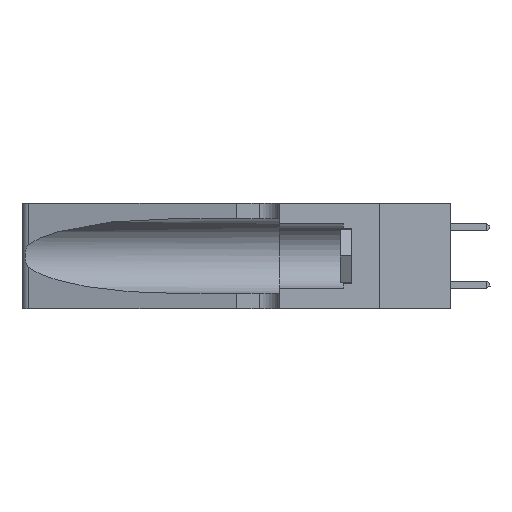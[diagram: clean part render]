
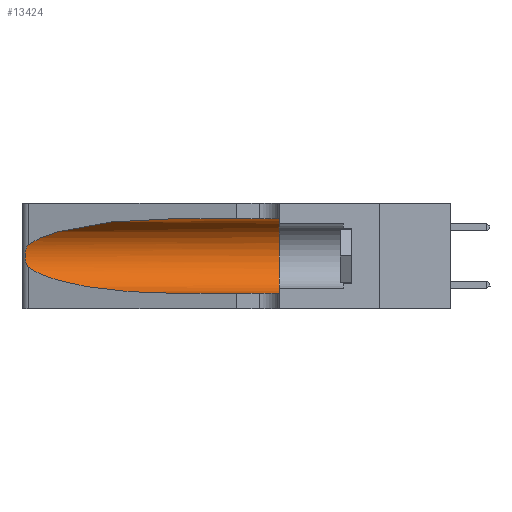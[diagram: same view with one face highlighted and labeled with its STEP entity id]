
A CAD part, left-side view. The second image highlights one B-rep face of the part: STEP entity #13424.
In plain terms, the highlighted cylindrical face has radius 3.308 mm (diameter 6.617 mm), a partial arc.
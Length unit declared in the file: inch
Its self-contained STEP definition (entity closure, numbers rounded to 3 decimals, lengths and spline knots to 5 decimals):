
#427 = CARTESIAN_POINT ( 'NONE',  ( 0.26018, 1.23835, 0.19895 ) ) ;
#2069 = ORIENTED_EDGE ( 'NONE', *, *, #15396, .F. ) ;
#2346 = CARTESIAN_POINT ( 'NONE',  ( 0.25487, 1.22718, 0.22369 ) ) ;
#3490 = CARTESIAN_POINT ( 'NONE',  ( 0.26075, 1.23896, 0.178 ) ) ;
#3949 = B_SPLINE_CURVE_WITH_KNOTS ( 'NONE', 3,
 ( #12381, #33062, #15370, #36014, #18378, #427, #21346, #3490, #24275, #6493, #27244, #9545, #30256, #12506 ),
 .UNSPECIFIED., .F., .F.,
 ( 4, 2, 2, 2, 2, 2, 4 ),
 ( 0., 0.00027, 0.00053, 0.00107, 0.0016, 0.00187, 0.00214 ),
 .UNSPECIFIED. ) ;
#4098 = CYLINDRICAL_SURFACE ( 'NONE', #31432, 0.13025 ) ;
#5398 = DIRECTION ( 'NONE',  ( 0., -1., 0. ) ) ;
#6035 = CARTESIAN_POINT ( 'NONE',  ( 0.18966, 0.96281, 0.05475 ) ) ;
#6493 = CARTESIAN_POINT ( 'NONE',  ( 0.25856, 1.23593, 0.16098 ) ) ;
#9225 = AXIS2_PLACEMENT_3D ( 'NONE', #27872, #10150, #30862 ) ;
#9545 = CARTESIAN_POINT ( 'NONE',  ( 0.25639, 1.23186, 0.15144 ) ) ;
#9634 = DIRECTION ( 'NONE',  ( 0., -1., 0. ) ) ;
#10150 = DIRECTION ( 'NONE',  ( 0., 1., 0. ) ) ;
#10249 = CARTESIAN_POINT ( 'NONE',  ( 0.1305, 0.35, 0.31525 ) ) ;
#10934 = CARTESIAN_POINT ( 'NONE',  ( 0.25487, 1.22718, 0.14631 ) ) ;
#12345 = ORIENTED_EDGE ( 'NONE', *, *, #25570, .T. ) ;
#12381 = CARTESIAN_POINT ( 'NONE',  ( 0.25487, 1.22718, 0.22369 ) ) ;
#12506 = CARTESIAN_POINT ( 'NONE',  ( 0.25487, 1.22718, 0.14631 ) ) ;
#13282 = VERTEX_POINT ( 'NONE', #10934 ) ;
#13424 = ADVANCED_FACE ( 'NONE', ( #27826 ), #4098, .F. ) ;
#13520 = LINE ( 'NONE', #27332, #29266 ) ;
#14432 = CARTESIAN_POINT ( 'NONE',  ( 0.1305, 1.61858, 0.185 ) ) ;
#14441 = DIRECTION ( 'NONE',  ( 0., -1., 0. ) ) ;
#14915 = CARTESIAN_POINT ( 'NONE',  ( 0.25487, 1.22718, 0.14631 ) ) ;
#15184 = VECTOR ( 'NONE', #14441, 39.37008 ) ;
#15370 = CARTESIAN_POINT ( 'NONE',  ( 0.25639, 1.23184, 0.21858 ) ) ;
#15396 = EDGE_CURVE ( 'NONE', #36557, #24557, #30006, .T. ) ;
#16826 = VERTEX_POINT ( 'NONE', #26480 ) ;
#16879 = CARTESIAN_POINT ( 'NONE',  ( 0.25487, 1.22718, 0.22369 ) ) ;
#17233 = CARTESIAN_POINT ( 'NONE',  ( 0.18966, 0.96281, 0.31525 ) ) ;
#17475 = ORIENTED_EDGE ( 'NONE', *, *, #31142, .T. ) ;
#17672 = CARTESIAN_POINT ( 'NONE',  ( 0.1305, 0.72297, 0.31525 ) ) ;
#17927 = CARTESIAN_POINT ( 'NONE',  ( 0.2373, 1.15595, 0.08982 ) ) ;
#18093 = CIRCLE ( 'NONE', #9225, 0.13025 ) ;
#18378 = CARTESIAN_POINT ( 'NONE',  ( 0.25854, 1.2359, 0.20912 ) ) ;
#20234 = CARTESIAN_POINT ( 'NONE',  ( 0.2373, 1.15595, 0.28018 ) ) ;
#21346 = CARTESIAN_POINT ( 'NONE',  ( 0.26075, 1.23896, 0.19203 ) ) ;
#23474 = ORIENTED_EDGE ( 'NONE', *, *, #36208, .F. ) ;
#23916 = ORIENTED_EDGE ( 'NONE', *, *, #31673, .T. ) ;
#24275 = CARTESIAN_POINT ( 'NONE',  ( 0.26017, 1.23833, 0.17102 ) ) ;
#24557 = VERTEX_POINT ( 'NONE', #10249 ) ;
#25570 = EDGE_CURVE ( 'NONE', #30898, #13282, #3949, .T. ) ;
#25694 = VERTEX_POINT ( 'NONE', #30759 ) ;
#26480 = CARTESIAN_POINT ( 'NONE',  ( 0.1305, 0.35, 0.05475 ) ) ;
#26792 = CARTESIAN_POINT ( 'NONE',  ( 0.1305, 0.72297, 0.05475 ) ) ;
#27244 = CARTESIAN_POINT ( 'NONE',  ( 0.25789, 1.23486, 0.15765 ) ) ;
#27266 = EDGE_CURVE ( 'NONE', #25694, #16826, #13520, .T. ) ;
#27332 = CARTESIAN_POINT ( 'NONE',  ( 0.1305, 1.61858, 0.05475 ) ) ;
#27826 = FACE_OUTER_BOUND ( 'NONE', #36133, .T. ) ;
#27872 = CARTESIAN_POINT ( 'NONE',  ( 0.1305, 0.35, 0.185 ) ) ;
#28980 = CARTESIAN_POINT ( 'NONE',  ( 0.1305, 0.72297, 0.31525 ) ) ;
#28998 =( BOUNDED_CURVE ( )  B_SPLINE_CURVE ( 3, ( #14915, #17927, #6035, #26792 ),
 .UNSPECIFIED., .F., .T. ) 
 B_SPLINE_CURVE_WITH_KNOTS ( ( 4, 4 ),
 ( 3.44316, 4.71239 ),
 .UNSPECIFIED. ) 
 CURVE ( )  GEOMETRIC_REPRESENTATION_ITEM ( )  RATIONAL_B_SPLINE_CURVE ( ( 1., 0.87, 0.87, 1. ) ) 
 REPRESENTATION_ITEM ( '' )  );
#29266 = VECTOR ( 'NONE', #9634, 39.37008 ) ;
#29945 = ORIENTED_EDGE ( 'NONE', *, *, #27266, .T. ) ;
#30006 = LINE ( 'NONE', #32159, #15184 ) ;
#30256 = CARTESIAN_POINT ( 'NONE',  ( 0.25555, 1.22993, 0.14849 ) ) ;
#30759 = CARTESIAN_POINT ( 'NONE',  ( 0.1305, 0.72297, 0.05475 ) ) ;
#30862 = DIRECTION ( 'NONE',  ( 0., 0., 1. ) ) ;
#30898 = VERTEX_POINT ( 'NONE', #16879 ) ;
#31142 = EDGE_CURVE ( 'NONE', #13282, #25694, #28998, .T. ) ;
#31432 = AXIS2_PLACEMENT_3D ( 'NONE', #14432, #5398, #32147 ) ;
#31673 = EDGE_CURVE ( 'NONE', #36557, #30898, #36507, .T. ) ;
#32147 = DIRECTION ( 'NONE',  ( 0., 0., -1. ) ) ;
#32159 = CARTESIAN_POINT ( 'NONE',  ( 0.1305, 1.61858, 0.31525 ) ) ;
#33062 = CARTESIAN_POINT ( 'NONE',  ( 0.25555, 1.22994, 0.2215 ) ) ;
#36014 = CARTESIAN_POINT ( 'NONE',  ( 0.25787, 1.23484, 0.2124 ) ) ;
#36133 = EDGE_LOOP ( 'NONE', ( #23916, #12345, #17475, #29945, #23474, #2069 ) ) ;
#36208 = EDGE_CURVE ( 'NONE', #24557, #16826, #18093, .T. ) ;
#36507 =( BOUNDED_CURVE ( )  B_SPLINE_CURVE ( 3, ( #28980, #17233, #20234, #2346 ),
 .UNSPECIFIED., .F., .T. ) 
 B_SPLINE_CURVE_WITH_KNOTS ( ( 4, 4 ),
 ( 1.5708, 2.84003 ),
 .UNSPECIFIED. ) 
 CURVE ( )  GEOMETRIC_REPRESENTATION_ITEM ( )  RATIONAL_B_SPLINE_CURVE ( ( 1., 0.87, 0.87, 1. ) ) 
 REPRESENTATION_ITEM ( '' )  );
#36557 = VERTEX_POINT ( 'NONE', #17672 ) ;
